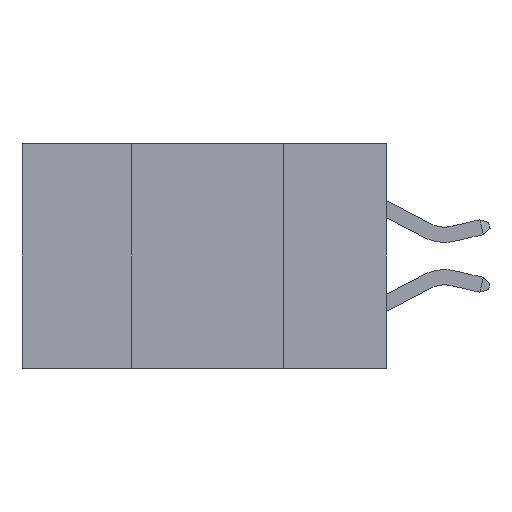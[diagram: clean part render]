
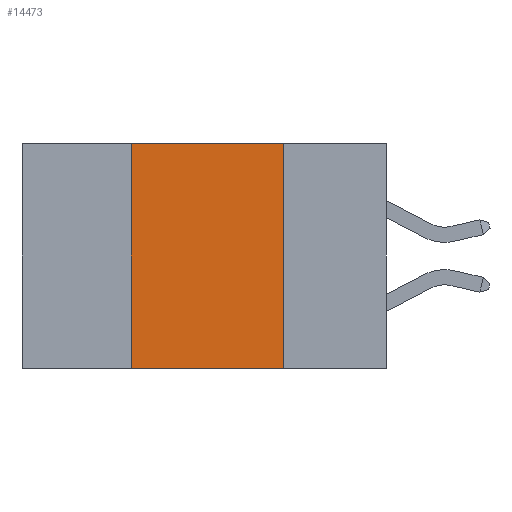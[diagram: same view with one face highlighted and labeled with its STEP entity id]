
A CAD part, left-side view. The second image highlights one B-rep face of the part: STEP entity #14473.
In plain terms, the highlighted planar face has unit normal (-1, 0, 0).
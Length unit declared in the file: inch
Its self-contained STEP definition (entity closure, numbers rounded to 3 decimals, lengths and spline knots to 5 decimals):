
#66 = AXIS2_PLACEMENT_3D ( 'NONE', #15385, #3034, #16849 ) ;
#440 = LINE ( 'NONE', #15575, #4966 ) ;
#1595 = CARTESIAN_POINT ( 'NONE',  ( 0., 0.42, -0.37 ) ) ;
#2408 = DIRECTION ( 'NONE',  ( 0., 0., 1. ) ) ;
#2736 = VERTEX_POINT ( 'NONE', #14271 ) ;
#3034 = DIRECTION ( 'NONE',  ( 1., 0., 0. ) ) ;
#3241 = LINE ( 'NONE', #9102, #7042 ) ;
#3280 = EDGE_CURVE ( 'NONE', #15732, #6351, #440, .T. ) ;
#3557 = EDGE_CURVE ( 'NONE', #15732, #2736, #9150, .T. ) ;
#4966 = VECTOR ( 'NONE', #12824, 39.37008 ) ;
#5292 = EDGE_LOOP ( 'NONE', ( #7652, #7178, #9223, #10390 ) ) ;
#5654 = EDGE_CURVE ( 'NONE', #17633, #6351, #11703, .T. ) ;
#6351 = VERTEX_POINT ( 'NONE', #13743 ) ;
#6453 = DIRECTION ( 'NONE',  ( 0., -1., 0. ) ) ;
#6542 = EDGE_CURVE ( 'NONE', #2736, #17633, #3241, .T. ) ;
#6950 = CARTESIAN_POINT ( 'NONE',  ( 0., 0.17, 0. ) ) ;
#7042 = VECTOR ( 'NONE', #6453, 39.37008 ) ;
#7178 = ORIENTED_EDGE ( 'NONE', *, *, #6542, .F. ) ;
#7652 = ORIENTED_EDGE ( 'NONE', *, *, #5654, .F. ) ;
#9102 = CARTESIAN_POINT ( 'NONE',  ( 0., 0.6, 0. ) ) ;
#9150 = LINE ( 'NONE', #17657, #14827 ) ;
#9223 = ORIENTED_EDGE ( 'NONE', *, *, #3557, .F. ) ;
#10390 = ORIENTED_EDGE ( 'NONE', *, *, #3280, .T. ) ;
#10519 = VECTOR ( 'NONE', #14611, 39.37008 ) ;
#11703 = LINE ( 'NONE', #17517, #10519 ) ;
#12654 = PLANE ( 'NONE',  #66 ) ;
#12824 = DIRECTION ( 'NONE',  ( 0., -1., 0. ) ) ;
#13743 = CARTESIAN_POINT ( 'NONE',  ( 0., 0.17, -0.37 ) ) ;
#14271 = CARTESIAN_POINT ( 'NONE',  ( 0., 0.42, 0. ) ) ;
#14473 = ADVANCED_FACE ( 'NONE', ( #16584 ), #12654, .F. ) ;
#14611 = DIRECTION ( 'NONE',  ( 0., 0., -1. ) ) ;
#14827 = VECTOR ( 'NONE', #2408, 39.37008 ) ;
#15385 = CARTESIAN_POINT ( 'NONE',  ( 0., 0.6, 0. ) ) ;
#15575 = CARTESIAN_POINT ( 'NONE',  ( 0., 0.6, -0.37 ) ) ;
#15732 = VERTEX_POINT ( 'NONE', #1595 ) ;
#16584 = FACE_OUTER_BOUND ( 'NONE', #5292, .T. ) ;
#16849 = DIRECTION ( 'NONE',  ( 0., 0., -1. ) ) ;
#17517 = CARTESIAN_POINT ( 'NONE',  ( 0., 0.17, -0.37 ) ) ;
#17633 = VERTEX_POINT ( 'NONE', #6950 ) ;
#17657 = CARTESIAN_POINT ( 'NONE',  ( 0., 0.42, -0.37 ) ) ;
